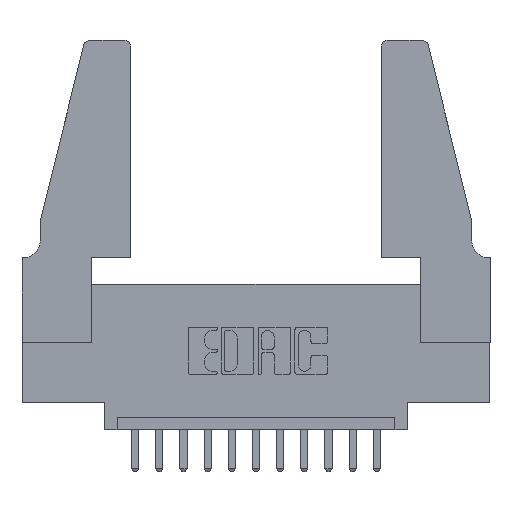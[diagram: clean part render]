
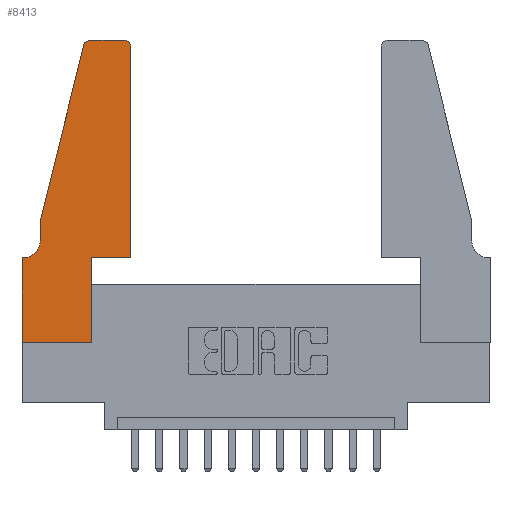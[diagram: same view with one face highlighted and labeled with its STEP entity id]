
A CAD part, top view. The second image highlights one B-rep face of the part: STEP entity #8413.
In plain terms, the highlighted planar face has unit normal (0, 0, 1).
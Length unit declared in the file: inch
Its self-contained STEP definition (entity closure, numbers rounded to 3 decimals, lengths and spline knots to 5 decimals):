
#302 = EDGE_CURVE ( 'NONE', #11718, #11859, #3004, .T. ) ;
#590 = DIRECTION ( 'NONE',  ( 0., 1., 0. ) ) ;
#1048 = CARTESIAN_POINT ( 'NONE',  ( 0.4205, 1.22, 0.37 ) ) ;
#1053 = ORIENTED_EDGE ( 'NONE', *, *, #14677, .T. ) ;
#1173 = VERTEX_POINT ( 'NONE', #11259 ) ;
#1308 = VERTEX_POINT ( 'NONE', #10428 ) ;
#1330 = CARTESIAN_POINT ( 'NONE',  ( 0.4505, 0.35, 0.37 ) ) ;
#1354 = LINE ( 'NONE', #13229, #2952 ) ;
#1417 = ORIENTED_EDGE ( 'NONE', *, *, #4917, .T. ) ;
#1798 = DIRECTION ( 'NONE',  ( -1., 0., 0. ) ) ;
#1829 = DIRECTION ( 'NONE',  ( 1., 0., 0. ) ) ;
#1917 = CARTESIAN_POINT ( 'NONE',  ( 0., 0., 0.37 ) ) ;
#1957 = AXIS2_PLACEMENT_3D ( 'NONE', #1048, #2095, #12281 ) ;
#1969 = VECTOR ( 'NONE', #10039, 39.37008 ) ;
#2003 = VERTEX_POINT ( 'NONE', #13867 ) ;
#2095 = DIRECTION ( 'NONE',  ( 0., 0., 1. ) ) ;
#2284 = VECTOR ( 'NONE', #6982, 39.37008 ) ;
#2376 = PLANE ( 'NONE',  #4726 ) ;
#2544 = LINE ( 'NONE', #1917, #2899 ) ;
#2645 = CARTESIAN_POINT ( 'NONE',  ( 0.284, 1.22, 0.37 ) ) ;
#2899 = VECTOR ( 'NONE', #9933, 39.37008 ) ;
#2952 = VECTOR ( 'NONE', #1798, 39.37008 ) ;
#3004 = CIRCLE ( 'NONE', #5719, 0.07 ) ;
#3619 = DIRECTION ( 'NONE',  ( 0., -1., 0. ) ) ;
#3778 = CARTESIAN_POINT ( 'NONE',  ( 0.0055, 0.42, 0.37 ) ) ;
#3959 = VECTOR ( 'NONE', #3619, 39.37008 ) ;
#3962 = CARTESIAN_POINT ( 'NONE',  ( 0.2865, 0.35, 0.37 ) ) ;
#4088 = EDGE_CURVE ( 'NONE', #9193, #9489, #7113, .T. ) ;
#4195 = CARTESIAN_POINT ( 'NONE',  ( 0.284, 1.25, 0.37 ) ) ;
#4264 = EDGE_LOOP ( 'NONE', ( #1417, #13619, #14556, #8246, #6580, #10120, #10105, #1053, #5481, #13482, #7744, #9609 ) ) ;
#4440 = LINE ( 'NONE', #1330, #2284 ) ;
#4474 = DIRECTION ( 'NONE',  ( 0., -1., 0. ) ) ;
#4726 = AXIS2_PLACEMENT_3D ( 'NONE', #14433, #10876, #1829 ) ;
#4847 = CIRCLE ( 'NONE', #6208, 0.03 ) ;
#4914 = DIRECTION ( 'NONE',  ( 0., 0., -1. ) ) ;
#4917 = EDGE_CURVE ( 'NONE', #10031, #11805, #1354, .T. ) ;
#4937 = VECTOR ( 'NONE', #590, 39.37008 ) ;
#5016 = CARTESIAN_POINT ( 'NONE',  ( 0.4505, 1.22, 0.37 ) ) ;
#5481 = ORIENTED_EDGE ( 'NONE', *, *, #4088, .T. ) ;
#5617 = CIRCLE ( 'NONE', #1957, 0.03 ) ;
#5719 = AXIS2_PLACEMENT_3D ( 'NONE', #3778, #4914, #8331 ) ;
#6208 = AXIS2_PLACEMENT_3D ( 'NONE', #2645, #8407, #11821 ) ;
#6211 = LINE ( 'NONE', #6749, #14676 ) ;
#6232 = CARTESIAN_POINT ( 'NONE',  ( 0.2865, 0., 0.37 ) ) ;
#6243 = CARTESIAN_POINT ( 'NONE',  ( 0.2865, 0.35, 0.37 ) ) ;
#6580 = ORIENTED_EDGE ( 'NONE', *, *, #302, .T. ) ;
#6690 = VERTEX_POINT ( 'NONE', #5016 ) ;
#6749 = CARTESIAN_POINT ( 'NONE',  ( 0.0755, 0.5, 0.37 ) ) ;
#6851 = EDGE_CURVE ( 'NONE', #6690, #10031, #5617, .T. ) ;
#6982 = DIRECTION ( 'NONE',  ( 0., 1., 0. ) ) ;
#7113 = LINE ( 'NONE', #3962, #4937 ) ;
#7194 = EDGE_CURVE ( 'NONE', #12778, #14711, #14401, .T. ) ;
#7661 = EDGE_CURVE ( 'NONE', #1308, #11718, #6211, .T. ) ;
#7721 = VECTOR ( 'NONE', #10526, 39.37008 ) ;
#7744 = ORIENTED_EDGE ( 'NONE', *, *, #13592, .T. ) ;
#8163 = FACE_OUTER_BOUND ( 'NONE', #4264, .T. ) ;
#8246 = ORIENTED_EDGE ( 'NONE', *, *, #7661, .T. ) ;
#8331 = DIRECTION ( 'NONE',  ( -1., 0., 0. ) ) ;
#8407 = DIRECTION ( 'NONE',  ( 0., 0., 1. ) ) ;
#8413 = ADVANCED_FACE ( 'NONE', ( #8163 ), #2376, .T. ) ;
#8485 = CARTESIAN_POINT ( 'NONE',  ( 0.0755, 0.42, 0.37 ) ) ;
#8784 = LINE ( 'NONE', #12489, #1969 ) ;
#9193 = VERTEX_POINT ( 'NONE', #6232 ) ;
#9489 = VERTEX_POINT ( 'NONE', #6243 ) ;
#9545 = DIRECTION ( 'NONE',  ( -0.239, -0.971, 0. ) ) ;
#9589 = CARTESIAN_POINT ( 'NONE',  ( 0.4205, 1.25, 0.37 ) ) ;
#9609 = ORIENTED_EDGE ( 'NONE', *, *, #6851, .T. ) ;
#9871 = LINE ( 'NONE', #13987, #7721 ) ;
#9933 = DIRECTION ( 'NONE',  ( 1., 0., 0. ) ) ;
#10031 = VERTEX_POINT ( 'NONE', #9589 ) ;
#10039 = DIRECTION ( 'NONE',  ( 1., 0., 0. ) ) ;
#10105 = ORIENTED_EDGE ( 'NONE', *, *, #7194, .T. ) ;
#10120 = ORIENTED_EDGE ( 'NONE', *, *, #11185, .T. ) ;
#10428 = CARTESIAN_POINT ( 'NONE',  ( 0.0755, 0.5, 0.37 ) ) ;
#10504 = EDGE_CURVE ( 'NONE', #11805, #2003, #4847, .T. ) ;
#10526 = DIRECTION ( 'NONE',  ( -1., 0., 0. ) ) ;
#10876 = DIRECTION ( 'NONE',  ( 0., 0., 1. ) ) ;
#11185 = EDGE_CURVE ( 'NONE', #11859, #12778, #9871, .T. ) ;
#11259 = CARTESIAN_POINT ( 'NONE',  ( 0.4505, 0.35, 0.37 ) ) ;
#11291 = LINE ( 'NONE', #11904, #13280 ) ;
#11652 = EDGE_CURVE ( 'NONE', #2003, #1308, #11291, .T. ) ;
#11718 = VERTEX_POINT ( 'NONE', #8485 ) ;
#11805 = VERTEX_POINT ( 'NONE', #4195 ) ;
#11821 = DIRECTION ( 'NONE',  ( 1., 0., 0. ) ) ;
#11859 = VERTEX_POINT ( 'NONE', #12374 ) ;
#11904 = CARTESIAN_POINT ( 'NONE',  ( 0.0755, 0.5, 0.37 ) ) ;
#12063 = CARTESIAN_POINT ( 'NONE',  ( 0., 0.35, 0.37 ) ) ;
#12281 = DIRECTION ( 'NONE',  ( 1., 0., 0. ) ) ;
#12365 = EDGE_CURVE ( 'NONE', #9489, #1173, #8784, .T. ) ;
#12374 = CARTESIAN_POINT ( 'NONE',  ( 0.0055, 0.35, 0.37 ) ) ;
#12377 = CARTESIAN_POINT ( 'NONE',  ( 0., 0., 0.37 ) ) ;
#12489 = CARTESIAN_POINT ( 'NONE',  ( 0.4505, 0.35, 0.37 ) ) ;
#12778 = VERTEX_POINT ( 'NONE', #12063 ) ;
#13229 = CARTESIAN_POINT ( 'NONE',  ( 0.2605, 1.25, 0.37 ) ) ;
#13280 = VECTOR ( 'NONE', #9545, 39.37008 ) ;
#13482 = ORIENTED_EDGE ( 'NONE', *, *, #12365, .T. ) ;
#13592 = EDGE_CURVE ( 'NONE', #1173, #6690, #4440, .T. ) ;
#13619 = ORIENTED_EDGE ( 'NONE', *, *, #10504, .T. ) ;
#13867 = CARTESIAN_POINT ( 'NONE',  ( 0.25487, 1.22718, 0.37 ) ) ;
#13987 = CARTESIAN_POINT ( 'NONE',  ( 0.0755, 0.35, 0.37 ) ) ;
#14401 = LINE ( 'NONE', #12377, #3959 ) ;
#14433 = CARTESIAN_POINT ( 'NONE',  ( 0., 0.35, 0.37 ) ) ;
#14556 = ORIENTED_EDGE ( 'NONE', *, *, #11652, .T. ) ;
#14676 = VECTOR ( 'NONE', #4474, 39.37008 ) ;
#14677 = EDGE_CURVE ( 'NONE', #14711, #9193, #2544, .T. ) ;
#14711 = VERTEX_POINT ( 'NONE', #14883 ) ;
#14883 = CARTESIAN_POINT ( 'NONE',  ( 0., 0., 0.37 ) ) ;
